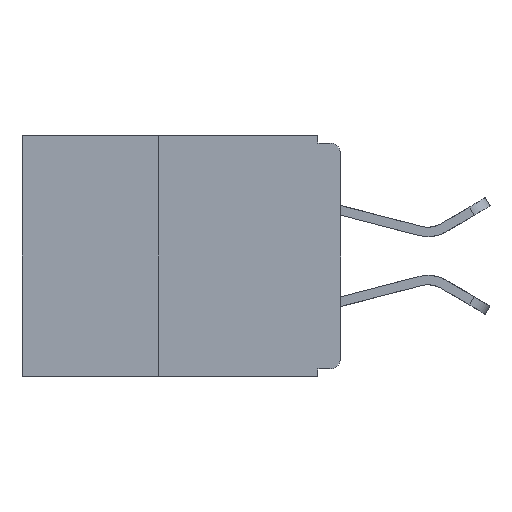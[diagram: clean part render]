
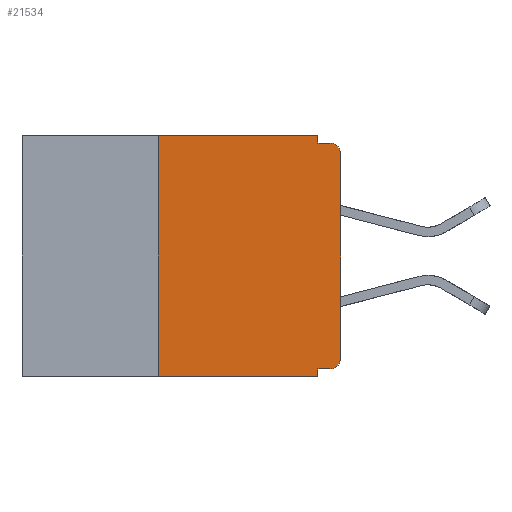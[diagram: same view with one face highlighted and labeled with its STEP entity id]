
A CAD part, left-side view. The second image highlights one B-rep face of the part: STEP entity #21534.
In plain terms, the highlighted planar face has unit normal (-1, 0, 0).
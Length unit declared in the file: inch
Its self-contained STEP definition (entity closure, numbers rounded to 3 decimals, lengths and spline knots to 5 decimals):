
#15 = CARTESIAN_POINT ( 'NONE',  ( 0., 0.031, 0. ) ) ;
#16 = DIRECTION ( 'NONE',  ( 0., 0., 1. ) ) ;
#27 = LINE ( 'NONE', #17962, #19644 ) ;
#342 = CARTESIAN_POINT ( 'NONE',  ( 0., 0.25, -0.33 ) ) ;
#596 = CARTESIAN_POINT ( 'NONE',  ( 0., 0.015, -0.305 ) ) ;
#997 = CARTESIAN_POINT ( 'NONE',  ( 0., 0.437, 0. ) ) ;
#1020 = VECTOR ( 'NONE', #22125, 39.37008 ) ;
#2132 = EDGE_LOOP ( 'NONE', ( #12496, #22731, #5487, #4683, #14701, #16362, #11688, #10279, #19340, #13812 ) ) ;
#2518 = VECTOR ( 'NONE', #11830, 39.37008 ) ;
#2535 = DIRECTION ( 'NONE',  ( 0., 0., -1. ) ) ;
#2918 = DIRECTION ( 'NONE',  ( 0., -1., 0. ) ) ;
#3304 = DIRECTION ( 'NONE',  ( -1., 0., 0. ) ) ;
#4375 = LINE ( 'NONE', #342, #8908 ) ;
#4683 = ORIENTED_EDGE ( 'NONE', *, *, #11284, .F. ) ;
#4900 = CIRCLE ( 'NONE', #9578, 0.015 ) ;
#5487 = ORIENTED_EDGE ( 'NONE', *, *, #18927, .F. ) ;
#5697 = EDGE_CURVE ( 'NONE', #12770, #17010, #13099, .T. ) ;
#6319 = EDGE_CURVE ( 'NONE', #12770, #13042, #4375, .T. ) ;
#6342 = DIRECTION ( 'NONE',  ( 0., 0., -1. ) ) ;
#7152 = CARTESIAN_POINT ( 'NONE',  ( 0., 0., 0. ) ) ;
#7245 = LINE ( 'NONE', #23442, #11754 ) ;
#7274 = PLANE ( 'NONE',  #13942 ) ;
#7536 = DIRECTION ( 'NONE',  ( 0., -1., 0. ) ) ;
#7731 = EDGE_CURVE ( 'NONE', #24270, #11654, #8237, .T. ) ;
#7867 = CARTESIAN_POINT ( 'NONE',  ( 0., 0.437, -0.33 ) ) ;
#8106 = EDGE_CURVE ( 'NONE', #9832, #11458, #4900, .T. ) ;
#8237 = CIRCLE ( 'NONE', #8762, 0.015 ) ;
#8762 = AXIS2_PLACEMENT_3D ( 'NONE', #14768, #3304, #16661 ) ;
#8908 = VECTOR ( 'NONE', #16, 39.37008 ) ;
#9180 = VECTOR ( 'NONE', #2918, 39.37008 ) ;
#9219 = DIRECTION ( 'NONE',  ( 0., 0., -1. ) ) ;
#9440 = VERTEX_POINT ( 'NONE', #12146 ) ;
#9578 = AXIS2_PLACEMENT_3D ( 'NONE', #596, #14022, #2535 ) ;
#9832 = VERTEX_POINT ( 'NONE', #15339 ) ;
#10279 = ORIENTED_EDGE ( 'NONE', *, *, #19456, .F. ) ;
#10635 = CARTESIAN_POINT ( 'NONE',  ( 0., 0., -0.305 ) ) ;
#11284 = EDGE_CURVE ( 'NONE', #19837, #13093, #18679, .T. ) ;
#11458 = VERTEX_POINT ( 'NONE', #10635 ) ;
#11654 = VERTEX_POINT ( 'NONE', #22306 ) ;
#11688 = ORIENTED_EDGE ( 'NONE', *, *, #5697, .T. ) ;
#11754 = VECTOR ( 'NONE', #14281, 39.37008 ) ;
#11830 = DIRECTION ( 'NONE',  ( 0., 1., 0. ) ) ;
#12146 = CARTESIAN_POINT ( 'NONE',  ( 0., 0.031, -0.32 ) ) ;
#12496 = ORIENTED_EDGE ( 'NONE', *, *, #24283, .T. ) ;
#12718 = LINE ( 'NONE', #21101, #2518 ) ;
#12770 = VERTEX_POINT ( 'NONE', #20209 ) ;
#13042 = VERTEX_POINT ( 'NONE', #19141 ) ;
#13093 = VERTEX_POINT ( 'NONE', #15595 ) ;
#13099 = LINE ( 'NONE', #7867, #21784 ) ;
#13812 = ORIENTED_EDGE ( 'NONE', *, *, #8106, .T. ) ;
#13942 = AXIS2_PLACEMENT_3D ( 'NONE', #16734, #20442, #9219 ) ;
#14022 = DIRECTION ( 'NONE',  ( -1., 0., 0. ) ) ;
#14281 = DIRECTION ( 'NONE',  ( 0., 0., -1. ) ) ;
#14316 = VECTOR ( 'NONE', #6342, 39.37008 ) ;
#14701 = ORIENTED_EDGE ( 'NONE', *, *, #24153, .F. ) ;
#14768 = CARTESIAN_POINT ( 'NONE',  ( 0., 0.015, -0.025 ) ) ;
#15339 = CARTESIAN_POINT ( 'NONE',  ( 0., 0.015, -0.32 ) ) ;
#15595 = CARTESIAN_POINT ( 'NONE',  ( 0., 0.031, -0.01 ) ) ;
#15998 = CARTESIAN_POINT ( 'NONE',  ( 0., 0.031, -0.33 ) ) ;
#16362 = ORIENTED_EDGE ( 'NONE', *, *, #6319, .F. ) ;
#16661 = DIRECTION ( 'NONE',  ( 0., 0., -1. ) ) ;
#16734 = CARTESIAN_POINT ( 'NONE',  ( 0., 0.437, 0. ) ) ;
#16865 = EDGE_CURVE ( 'NONE', #9832, #9440, #12718, .T. ) ;
#17010 = VERTEX_POINT ( 'NONE', #15998 ) ;
#17683 = CARTESIAN_POINT ( 'NONE',  ( 0., 0.031, 0. ) ) ;
#17962 = CARTESIAN_POINT ( 'NONE',  ( 0., 0., -0.01 ) ) ;
#18444 = CARTESIAN_POINT ( 'NONE',  ( 0., 0., -0.025 ) ) ;
#18679 = LINE ( 'NONE', #17683, #14316 ) ;
#18927 = EDGE_CURVE ( 'NONE', #13093, #11654, #27, .T. ) ;
#19141 = CARTESIAN_POINT ( 'NONE',  ( 0., 0.25, 0. ) ) ;
#19340 = ORIENTED_EDGE ( 'NONE', *, *, #16865, .F. ) ;
#19456 = EDGE_CURVE ( 'NONE', #9440, #17010, #7245, .T. ) ;
#19644 = VECTOR ( 'NONE', #19817, 39.37008 ) ;
#19817 = DIRECTION ( 'NONE',  ( 0., -1., 0. ) ) ;
#19837 = VERTEX_POINT ( 'NONE', #15 ) ;
#20209 = CARTESIAN_POINT ( 'NONE',  ( 0., 0.25, -0.33 ) ) ;
#20442 = DIRECTION ( 'NONE',  ( 1., 0., 0. ) ) ;
#20612 = LINE ( 'NONE', #7152, #1020 ) ;
#21101 = CARTESIAN_POINT ( 'NONE',  ( 0., 0., -0.32 ) ) ;
#21534 = ADVANCED_FACE ( 'NONE', ( #22445 ), #7274, .F. ) ;
#21784 = VECTOR ( 'NONE', #7536, 39.37008 ) ;
#22125 = DIRECTION ( 'NONE',  ( 0., 0., 1. ) ) ;
#22306 = CARTESIAN_POINT ( 'NONE',  ( 0., 0.015, -0.01 ) ) ;
#22445 = FACE_OUTER_BOUND ( 'NONE', #2132, .T. ) ;
#22731 = ORIENTED_EDGE ( 'NONE', *, *, #7731, .T. ) ;
#23442 = CARTESIAN_POINT ( 'NONE',  ( 0., 0.031, -0.33 ) ) ;
#23986 = LINE ( 'NONE', #997, #9180 ) ;
#24153 = EDGE_CURVE ( 'NONE', #13042, #19837, #23986, .T. ) ;
#24270 = VERTEX_POINT ( 'NONE', #18444 ) ;
#24283 = EDGE_CURVE ( 'NONE', #11458, #24270, #20612, .T. ) ;
